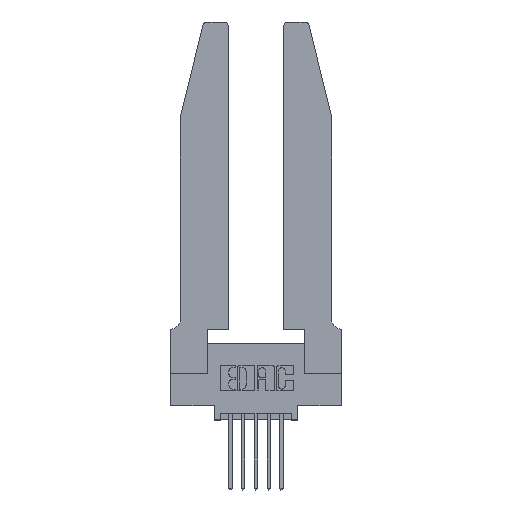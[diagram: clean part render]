
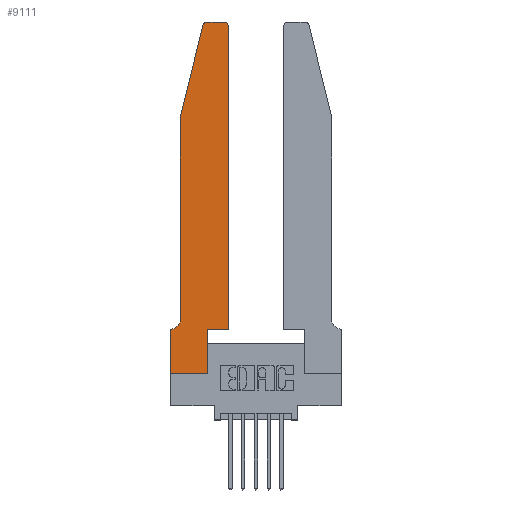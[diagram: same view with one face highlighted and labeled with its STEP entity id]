
A CAD part, top view. The second image highlights one B-rep face of the part: STEP entity #9111.
In plain terms, the highlighted planar face has unit normal (0, 0, 1).
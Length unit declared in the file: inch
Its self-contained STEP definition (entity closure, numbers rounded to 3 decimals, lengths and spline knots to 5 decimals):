
#187 = LINE ( 'NONE', #10863, #4742 ) ;
#456 = AXIS2_PLACEMENT_3D ( 'NONE', #10657, #3137, #12787 ) ;
#582 = CARTESIAN_POINT ( 'NONE',  ( 0.0755, 2., 0.37 ) ) ;
#744 = VERTEX_POINT ( 'NONE', #9548 ) ;
#787 = EDGE_CURVE ( 'NONE', #7021, #744, #8287, .T. ) ;
#1019 = CARTESIAN_POINT ( 'NONE',  ( 0.4505, 0.35, 0.37 ) ) ;
#1102 = CARTESIAN_POINT ( 'NONE',  ( 0.4505, 2.72, 0.37 ) ) ;
#1145 = DIRECTION ( 'NONE',  ( -1., 0., 0. ) ) ;
#1393 = CARTESIAN_POINT ( 'NONE',  ( 0.0755, 2., 0.37 ) ) ;
#1734 = LINE ( 'NONE', #13073, #9244 ) ;
#1843 = VECTOR ( 'NONE', #3552, 39.37008 ) ;
#1927 = VERTEX_POINT ( 'NONE', #4503 ) ;
#2144 = LINE ( 'NONE', #582, #7495 ) ;
#2296 = CIRCLE ( 'NONE', #456, 0.03 ) ;
#2368 = DIRECTION ( 'NONE',  ( 1., 0., 0. ) ) ;
#2417 = VERTEX_POINT ( 'NONE', #6186 ) ;
#2458 = FACE_OUTER_BOUND ( 'NONE', #8482, .T. ) ;
#2597 = EDGE_CURVE ( 'NONE', #6499, #10922, #1734, .T. ) ;
#2709 = LINE ( 'NONE', #5348, #10230 ) ;
#2752 = VECTOR ( 'NONE', #8545, 39.37008 ) ;
#3137 = DIRECTION ( 'NONE',  ( 0., 0., 1. ) ) ;
#3452 = EDGE_CURVE ( 'NONE', #2417, #12908, #187, .T. ) ;
#3552 = DIRECTION ( 'NONE',  ( 0., -1., 0. ) ) ;
#3840 = DIRECTION ( 'NONE',  ( -1., 0., 0. ) ) ;
#4031 = DIRECTION ( 'NONE',  ( 1., 0., 0. ) ) ;
#4233 = CARTESIAN_POINT ( 'NONE',  ( 0.25487, 2.72718, 0.37 ) ) ;
#4337 = DIRECTION ( 'NONE',  ( 0., 1., 0. ) ) ;
#4503 = CARTESIAN_POINT ( 'NONE',  ( 0.2865, 0.35, 0.37 ) ) ;
#4598 = ORIENTED_EDGE ( 'NONE', *, *, #13793, .T. ) ;
#4742 = VECTOR ( 'NONE', #1145, 39.37008 ) ;
#4836 = CARTESIAN_POINT ( 'NONE',  ( 0.0755, 0.42, 0.37 ) ) ;
#5018 = DIRECTION ( 'NONE',  ( 0., 1., 0. ) ) ;
#5314 = DIRECTION ( 'NONE',  ( -1., 0., 0. ) ) ;
#5341 = CARTESIAN_POINT ( 'NONE',  ( 0., 0., 0.37 ) ) ;
#5348 = CARTESIAN_POINT ( 'NONE',  ( 0.2865, 0.35, 0.37 ) ) ;
#5356 = DIRECTION ( 'NONE',  ( 0., 0., -1. ) ) ;
#5503 = LINE ( 'NONE', #10741, #6176 ) ;
#5535 = EDGE_CURVE ( 'NONE', #12449, #12281, #2144, .T. ) ;
#5666 = EDGE_CURVE ( 'NONE', #744, #10352, #13819, .T. ) ;
#5801 = ORIENTED_EDGE ( 'NONE', *, *, #7482, .T. ) ;
#5924 = AXIS2_PLACEMENT_3D ( 'NONE', #11669, #5356, #5314 ) ;
#6176 = VECTOR ( 'NONE', #7470, 39.37008 ) ;
#6186 = CARTESIAN_POINT ( 'NONE',  ( 0.0055, 0.35, 0.37 ) ) ;
#6408 = CARTESIAN_POINT ( 'NONE',  ( 0., 0.35, 0.37 ) ) ;
#6499 = VERTEX_POINT ( 'NONE', #8472 ) ;
#6695 = ORIENTED_EDGE ( 'NONE', *, *, #13754, .T. ) ;
#6729 = VECTOR ( 'NONE', #5018, 39.37008 ) ;
#6984 = ORIENTED_EDGE ( 'NONE', *, *, #787, .T. ) ;
#7021 = VERTEX_POINT ( 'NONE', #1102 ) ;
#7037 = DIRECTION ( 'NONE',  ( -0.239, -0.971, 0. ) ) ;
#7052 = ORIENTED_EDGE ( 'NONE', *, *, #5666, .T. ) ;
#7223 = CIRCLE ( 'NONE', #5924, 0.07 ) ;
#7470 = DIRECTION ( 'NONE',  ( 1., 0., 0. ) ) ;
#7482 = EDGE_CURVE ( 'NONE', #12281, #8260, #10363, .T. ) ;
#7495 = VECTOR ( 'NONE', #7037, 39.37008 ) ;
#7837 = AXIS2_PLACEMENT_3D ( 'NONE', #8778, #11874, #2368 ) ;
#7949 = ORIENTED_EDGE ( 'NONE', *, *, #5535, .T. ) ;
#7978 = VERTEX_POINT ( 'NONE', #1019 ) ;
#8205 = AXIS2_PLACEMENT_3D ( 'NONE', #6408, #10681, #9404 ) ;
#8260 = VERTEX_POINT ( 'NONE', #4836 ) ;
#8266 = LINE ( 'NONE', #5341, #2752 ) ;
#8287 = CIRCLE ( 'NONE', #7837, 0.03 ) ;
#8455 = CARTESIAN_POINT ( 'NONE',  ( 0.284, 2.75, 0.37 ) ) ;
#8472 = CARTESIAN_POINT ( 'NONE',  ( 0., 0., 0.37 ) ) ;
#8482 = EDGE_LOOP ( 'NONE', ( #7052, #6695, #7949, #5801, #8779, #11028, #13776, #12259, #10034, #4598, #8666, #6984 ) ) ;
#8545 = DIRECTION ( 'NONE',  ( 0., -1., 0. ) ) ;
#8666 = ORIENTED_EDGE ( 'NONE', *, *, #12915, .T. ) ;
#8778 = CARTESIAN_POINT ( 'NONE',  ( 0.4205, 2.72, 0.37 ) ) ;
#8779 = ORIENTED_EDGE ( 'NONE', *, *, #11828, .T. ) ;
#9111 = ADVANCED_FACE ( 'NONE', ( #2458 ), #11681, .T. ) ;
#9244 = VECTOR ( 'NONE', #4031, 39.37008 ) ;
#9404 = DIRECTION ( 'NONE',  ( 1., 0., 0. ) ) ;
#9548 = CARTESIAN_POINT ( 'NONE',  ( 0.4205, 2.75, 0.37 ) ) ;
#10034 = ORIENTED_EDGE ( 'NONE', *, *, #12372, .T. ) ;
#10230 = VECTOR ( 'NONE', #4337, 39.37008 ) ;
#10352 = VERTEX_POINT ( 'NONE', #8455 ) ;
#10363 = LINE ( 'NONE', #1393, #1843 ) ;
#10365 = EDGE_CURVE ( 'NONE', #12908, #6499, #8266, .T. ) ;
#10657 = CARTESIAN_POINT ( 'NONE',  ( 0.284, 2.72, 0.37 ) ) ;
#10681 = DIRECTION ( 'NONE',  ( 0., 0., 1. ) ) ;
#10741 = CARTESIAN_POINT ( 'NONE',  ( 0.4505, 0.35, 0.37 ) ) ;
#10744 = LINE ( 'NONE', #13321, #6729 ) ;
#10863 = CARTESIAN_POINT ( 'NONE',  ( 0.0755, 0.35, 0.37 ) ) ;
#10922 = VERTEX_POINT ( 'NONE', #12242 ) ;
#10995 = VECTOR ( 'NONE', #3840, 39.37008 ) ;
#11028 = ORIENTED_EDGE ( 'NONE', *, *, #3452, .T. ) ;
#11149 = CARTESIAN_POINT ( 'NONE',  ( 0.2605, 2.75, 0.37 ) ) ;
#11195 = CARTESIAN_POINT ( 'NONE',  ( 0., 0.35, 0.37 ) ) ;
#11344 = CARTESIAN_POINT ( 'NONE',  ( 0.0755, 2., 0.37 ) ) ;
#11669 = CARTESIAN_POINT ( 'NONE',  ( 0.0055, 0.42, 0.37 ) ) ;
#11681 = PLANE ( 'NONE',  #8205 ) ;
#11828 = EDGE_CURVE ( 'NONE', #8260, #2417, #7223, .T. ) ;
#11874 = DIRECTION ( 'NONE',  ( 0., 0., 1. ) ) ;
#12242 = CARTESIAN_POINT ( 'NONE',  ( 0.2865, 0., 0.37 ) ) ;
#12259 = ORIENTED_EDGE ( 'NONE', *, *, #2597, .T. ) ;
#12281 = VERTEX_POINT ( 'NONE', #11344 ) ;
#12372 = EDGE_CURVE ( 'NONE', #10922, #1927, #2709, .T. ) ;
#12449 = VERTEX_POINT ( 'NONE', #4233 ) ;
#12787 = DIRECTION ( 'NONE',  ( 1., 0., 0. ) ) ;
#12908 = VERTEX_POINT ( 'NONE', #11195 ) ;
#12915 = EDGE_CURVE ( 'NONE', #7978, #7021, #10744, .T. ) ;
#13073 = CARTESIAN_POINT ( 'NONE',  ( 0., 0., 0.37 ) ) ;
#13321 = CARTESIAN_POINT ( 'NONE',  ( 0.4505, 0.35, 0.37 ) ) ;
#13754 = EDGE_CURVE ( 'NONE', #10352, #12449, #2296, .T. ) ;
#13776 = ORIENTED_EDGE ( 'NONE', *, *, #10365, .T. ) ;
#13793 = EDGE_CURVE ( 'NONE', #1927, #7978, #5503, .T. ) ;
#13819 = LINE ( 'NONE', #11149, #10995 ) ;
